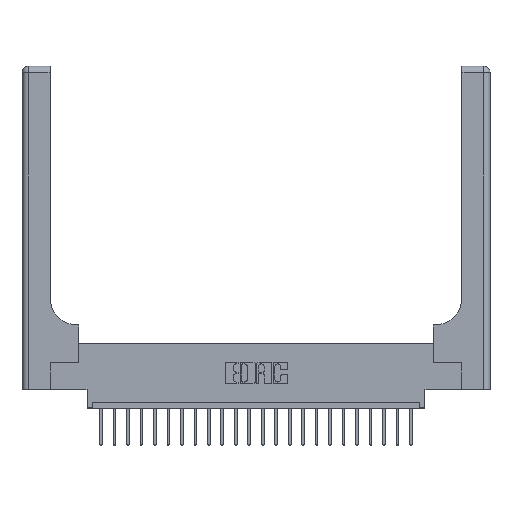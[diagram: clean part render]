
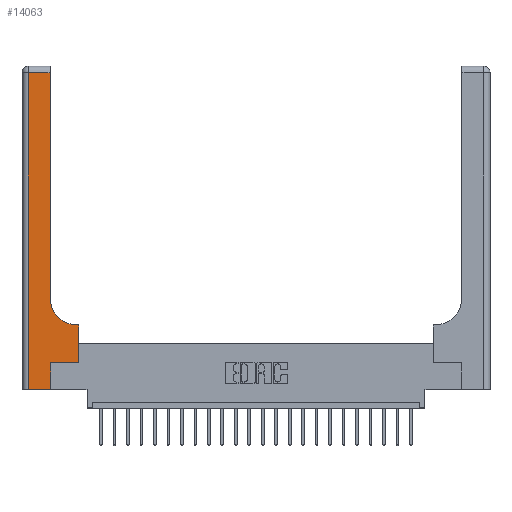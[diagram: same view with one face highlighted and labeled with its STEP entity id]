
A CAD part, top view. The second image highlights one B-rep face of the part: STEP entity #14063.
In plain terms, the highlighted planar face has unit normal (0, 0, 1).
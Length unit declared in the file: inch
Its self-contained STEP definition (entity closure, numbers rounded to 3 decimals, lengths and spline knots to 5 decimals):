
#21 = LINE ( 'NONE', #21114, #7138 ) ;
#135 = VECTOR ( 'NONE', #21837, 39.37008 ) ;
#310 = DIRECTION ( 'NONE',  ( -1., 0., 0. ) ) ;
#553 = VERTEX_POINT ( 'NONE', #16038 ) ;
#564 = CARTESIAN_POINT ( 'NONE',  ( 0.51, 0.6, 0.37 ) ) ;
#588 = EDGE_CURVE ( 'NONE', #16575, #8036, #2396, .T. ) ;
#986 = VECTOR ( 'NONE', #10609, 39.37008 ) ;
#1037 = FACE_OUTER_BOUND ( 'NONE', #21710, .T. ) ;
#1834 = CARTESIAN_POINT ( 'NONE',  ( 0.06, 0., 0.37 ) ) ;
#1861 = VERTEX_POINT ( 'NONE', #6982 ) ;
#1999 = CARTESIAN_POINT ( 'NONE',  ( 0., 3., 0.37 ) ) ;
#2396 = LINE ( 'NONE', #21169, #14427 ) ;
#2564 = CARTESIAN_POINT ( 'NONE',  ( 0.06, 3., 0.37 ) ) ;
#2592 = DIRECTION ( 'NONE',  ( 0., 0., -1. ) ) ;
#3154 = CARTESIAN_POINT ( 'NONE',  ( 0.06, 2.94, 0.37 ) ) ;
#3519 = VECTOR ( 'NONE', #8054, 39.37008 ) ;
#3585 = EDGE_CURVE ( 'NONE', #8036, #13327, #8338, .T. ) ;
#3666 = CARTESIAN_POINT ( 'NONE',  ( 0.528, 0.6, 0.37 ) ) ;
#3951 = PLANE ( 'NONE',  #19534 ) ;
#4278 = VERTEX_POINT ( 'NONE', #9736 ) ;
#4327 = VECTOR ( 'NONE', #8845, 39.37008 ) ;
#4534 = CARTESIAN_POINT ( 'NONE',  ( 0.265, 0., 0.37 ) ) ;
#5246 = VERTEX_POINT ( 'NONE', #1834 ) ;
#6716 = LINE ( 'NONE', #13539, #9708 ) ;
#6982 = CARTESIAN_POINT ( 'NONE',  ( 0.26, 2.94, 0.37 ) ) ;
#7138 = VECTOR ( 'NONE', #19242, 39.37008 ) ;
#7718 = LINE ( 'NONE', #4534, #12881 ) ;
#7877 = AXIS2_PLACEMENT_3D ( 'NONE', #11474, #2592, #13284 ) ;
#8036 = VERTEX_POINT ( 'NONE', #564 ) ;
#8054 = DIRECTION ( 'NONE',  ( 1., 0., 0. ) ) ;
#8338 = CIRCLE ( 'NONE', #7877, 0.25 ) ;
#8813 = EDGE_CURVE ( 'NONE', #17652, #5246, #9971, .T. ) ;
#8845 = DIRECTION ( 'NONE',  ( 0., 1., 0. ) ) ;
#8857 = DIRECTION ( 'NONE',  ( -1., 0., 0. ) ) ;
#8979 = LINE ( 'NONE', #17544, #4327 ) ;
#9708 = VECTOR ( 'NONE', #17060, 39.37008 ) ;
#9736 = CARTESIAN_POINT ( 'NONE',  ( 0.265, 0., 0.37 ) ) ;
#9971 = LINE ( 'NONE', #2564, #135 ) ;
#10257 = EDGE_CURVE ( 'NONE', #10279, #553, #21, .T. ) ;
#10279 = VERTEX_POINT ( 'NONE', #19010 ) ;
#10426 = ORIENTED_EDGE ( 'NONE', *, *, #15152, .T. ) ;
#10609 = DIRECTION ( 'NONE',  ( 0., 1., 0. ) ) ;
#11179 = EDGE_CURVE ( 'NONE', #4278, #10279, #7718, .T. ) ;
#11474 = CARTESIAN_POINT ( 'NONE',  ( 0.51, 0.85, 0.37 ) ) ;
#11608 = ORIENTED_EDGE ( 'NONE', *, *, #13680, .T. ) ;
#11927 = ORIENTED_EDGE ( 'NONE', *, *, #10257, .T. ) ;
#11993 = CARTESIAN_POINT ( 'NONE',  ( 0.26, 0.85, 0.37 ) ) ;
#12417 = ORIENTED_EDGE ( 'NONE', *, *, #11179, .T. ) ;
#12881 = VECTOR ( 'NONE', #18196, 39.37008 ) ;
#13284 = DIRECTION ( 'NONE',  ( 1., 0., 0. ) ) ;
#13327 = VERTEX_POINT ( 'NONE', #11993 ) ;
#13500 = ORIENTED_EDGE ( 'NONE', *, *, #3585, .T. ) ;
#13510 = EDGE_CURVE ( 'NONE', #553, #16575, #8979, .T. ) ;
#13539 = CARTESIAN_POINT ( 'NONE',  ( 0., 2.94, 0.37 ) ) ;
#13680 = EDGE_CURVE ( 'NONE', #5246, #4278, #21870, .T. ) ;
#14063 = ADVANCED_FACE ( 'NONE', ( #1037 ), #3951, .F. ) ;
#14427 = VECTOR ( 'NONE', #8857, 39.37008 ) ;
#14762 = ORIENTED_EDGE ( 'NONE', *, *, #13510, .T. ) ;
#15152 = EDGE_CURVE ( 'NONE', #13327, #1861, #17385, .T. ) ;
#16038 = CARTESIAN_POINT ( 'NONE',  ( 0.528, 0.25, 0.37 ) ) ;
#16575 = VERTEX_POINT ( 'NONE', #3666 ) ;
#16746 = ORIENTED_EDGE ( 'NONE', *, *, #20304, .T. ) ;
#17060 = DIRECTION ( 'NONE',  ( -1., 0., 0. ) ) ;
#17310 = CARTESIAN_POINT ( 'NONE',  ( 0.26, 3., 0.37 ) ) ;
#17385 = LINE ( 'NONE', #17310, #986 ) ;
#17544 = CARTESIAN_POINT ( 'NONE',  ( 0.528, 0.25, 0.37 ) ) ;
#17652 = VERTEX_POINT ( 'NONE', #3154 ) ;
#18196 = DIRECTION ( 'NONE',  ( 0., 1., 0. ) ) ;
#18411 = CARTESIAN_POINT ( 'NONE',  ( 0., 0., 0.37 ) ) ;
#18560 = ORIENTED_EDGE ( 'NONE', *, *, #588, .T. ) ;
#19010 = CARTESIAN_POINT ( 'NONE',  ( 0.265, 0.25, 0.37 ) ) ;
#19242 = DIRECTION ( 'NONE',  ( 1., 0., 0. ) ) ;
#19534 = AXIS2_PLACEMENT_3D ( 'NONE', #1999, #20757, #310 ) ;
#20304 = EDGE_CURVE ( 'NONE', #1861, #17652, #6716, .T. ) ;
#20757 = DIRECTION ( 'NONE',  ( 0., 0., -1. ) ) ;
#21114 = CARTESIAN_POINT ( 'NONE',  ( 0.265, 0.25, 0.37 ) ) ;
#21169 = CARTESIAN_POINT ( 'NONE',  ( 0.26, 0.6, 0.37 ) ) ;
#21710 = EDGE_LOOP ( 'NONE', ( #10426, #16746, #22155, #11608, #12417, #11927, #14762, #18560, #13500 ) ) ;
#21837 = DIRECTION ( 'NONE',  ( 0., -1., 0. ) ) ;
#21870 = LINE ( 'NONE', #18411, #3519 ) ;
#22155 = ORIENTED_EDGE ( 'NONE', *, *, #8813, .T. ) ;
